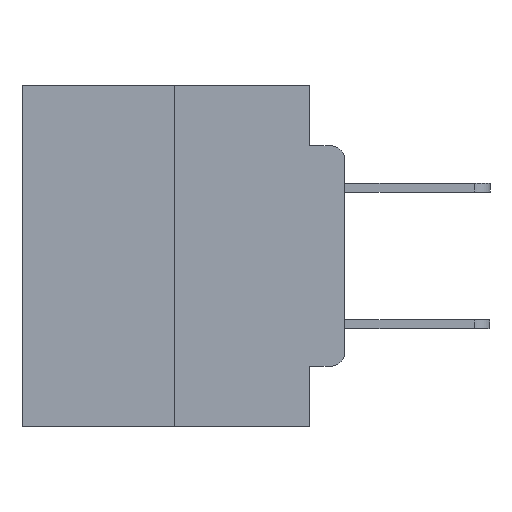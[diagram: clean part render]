
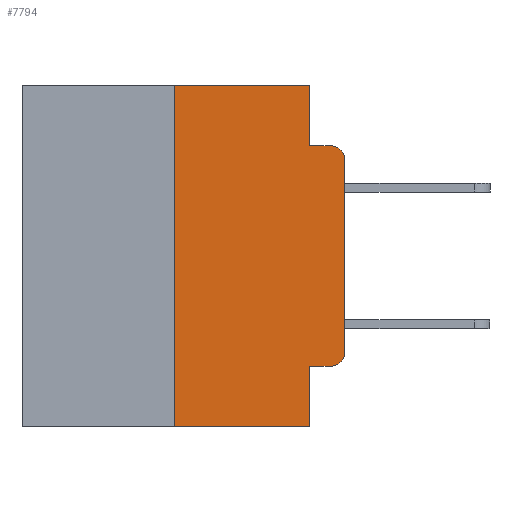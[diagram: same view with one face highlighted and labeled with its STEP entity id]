
A CAD part, left-side view. The second image highlights one B-rep face of the part: STEP entity #7794.
In plain terms, the highlighted planar face has unit normal (-1, 0, 0).
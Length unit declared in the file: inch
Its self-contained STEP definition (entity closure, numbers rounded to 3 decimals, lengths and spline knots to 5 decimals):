
#229 = VERTEX_POINT ( 'NONE', #24370 ) ;
#333 = DIRECTION ( 'NONE',  ( -1., 0., 0. ) ) ;
#425 = CARTESIAN_POINT ( 'NONE',  ( 0., 0.473, 0. ) ) ;
#692 = DIRECTION ( 'NONE',  ( -1., 0., 0. ) ) ;
#1464 = FACE_OUTER_BOUND ( 'NONE', #6110, .T. ) ;
#1516 = CARTESIAN_POINT ( 'NONE',  ( 0., 0.051, -0.0885 ) ) ;
#1519 = VERTEX_POINT ( 'NONE', #24135 ) ;
#2058 = ORIENTED_EDGE ( 'NONE', *, *, #5218, .F. ) ;
#2216 = VERTEX_POINT ( 'NONE', #14894 ) ;
#2325 = EDGE_CURVE ( 'NONE', #20849, #1519, #4652, .T. ) ;
#2396 = AXIS2_PLACEMENT_3D ( 'NONE', #13055, #333, #15138 ) ;
#3966 = LINE ( 'NONE', #7773, #14443 ) ;
#4499 = CARTESIAN_POINT ( 'NONE',  ( 0., 0.051, -0.4115 ) ) ;
#4652 = LINE ( 'NONE', #6540, #10197 ) ;
#5218 = EDGE_CURVE ( 'NONE', #9218, #19917, #16582, .T. ) ;
#5557 = VECTOR ( 'NONE', #22373, 39.37008 ) ;
#6054 = VECTOR ( 'NONE', #15220, 39.37008 ) ;
#6100 = CARTESIAN_POINT ( 'NONE',  ( 0., 0.473, 0. ) ) ;
#6110 = EDGE_LOOP ( 'NONE', ( #26407, #10629, #16791, #6409, #22850, #2058, #24161, #14549, #20001, #15845 ) ) ;
#6195 = DIRECTION ( 'NONE',  ( 0., 0., -1. ) ) ;
#6409 = ORIENTED_EDGE ( 'NONE', *, *, #2325, .F. ) ;
#6540 = CARTESIAN_POINT ( 'NONE',  ( 0., 0.051, 0. ) ) ;
#7129 = EDGE_CURVE ( 'NONE', #1519, #9947, #11082, .T. ) ;
#7773 = CARTESIAN_POINT ( 'NONE',  ( 0., 0.051, 0. ) ) ;
#7794 = ADVANCED_FACE ( 'NONE', ( #1464 ), #24679, .F. ) ;
#8178 = CARTESIAN_POINT ( 'NONE',  ( 0., 0.051, -0.4115 ) ) ;
#8709 = CARTESIAN_POINT ( 'NONE',  ( 0., 0.051, 0. ) ) ;
#9218 = VERTEX_POINT ( 'NONE', #23624 ) ;
#9471 = CARTESIAN_POINT ( 'NONE',  ( 0., 0., -0.1085 ) ) ;
#9864 = DIRECTION ( 'NONE',  ( 0., 0., -1. ) ) ;
#9947 = VERTEX_POINT ( 'NONE', #22607 ) ;
#10197 = VECTOR ( 'NONE', #10483, 39.37008 ) ;
#10483 = DIRECTION ( 'NONE',  ( 0., 0., -1. ) ) ;
#10629 = ORIENTED_EDGE ( 'NONE', *, *, #25618, .T. ) ;
#10925 = LINE ( 'NONE', #425, #6054 ) ;
#10948 = DIRECTION ( 'NONE',  ( 0., 0., 1. ) ) ;
#11082 = LINE ( 'NONE', #1516, #5557 ) ;
#11092 = LINE ( 'NONE', #16320, #15986 ) ;
#11131 = AXIS2_PLACEMENT_3D ( 'NONE', #6100, #18591, #6195 ) ;
#11850 = CARTESIAN_POINT ( 'NONE',  ( 0., 0.473, -0.5 ) ) ;
#12018 = EDGE_CURVE ( 'NONE', #229, #2216, #24056, .T. ) ;
#13055 = CARTESIAN_POINT ( 'NONE',  ( 0., 0.02, -0.3915 ) ) ;
#13382 = CARTESIAN_POINT ( 'NONE',  ( 0., 0.02, -0.1085 ) ) ;
#13975 = DIRECTION ( 'NONE',  ( 0., -1., 0. ) ) ;
#14443 = VECTOR ( 'NONE', #9864, 39.37008 ) ;
#14488 = CIRCLE ( 'NONE', #19791, 0.02 ) ;
#14549 = ORIENTED_EDGE ( 'NONE', *, *, #24588, .F. ) ;
#14894 = CARTESIAN_POINT ( 'NONE',  ( 0., 0., -0.3915 ) ) ;
#15100 = VECTOR ( 'NONE', #13975, 39.37008 ) ;
#15138 = DIRECTION ( 'NONE',  ( 0., 0., -1. ) ) ;
#15152 = CARTESIAN_POINT ( 'NONE',  ( 0., 0.25, 0. ) ) ;
#15220 = DIRECTION ( 'NONE',  ( 0., -1., 0. ) ) ;
#15232 = LINE ( 'NONE', #8178, #24816 ) ;
#15352 = EDGE_CURVE ( 'NONE', #17832, #229, #15232, .T. ) ;
#15465 = DIRECTION ( 'NONE',  ( 0., 0., -1. ) ) ;
#15573 = CARTESIAN_POINT ( 'NONE',  ( 0., 0.051, -0.5 ) ) ;
#15845 = ORIENTED_EDGE ( 'NONE', *, *, #12018, .T. ) ;
#15986 = VECTOR ( 'NONE', #22479, 39.37008 ) ;
#16320 = CARTESIAN_POINT ( 'NONE',  ( 0., 0., 0. ) ) ;
#16582 = LINE ( 'NONE', #15152, #21385 ) ;
#16791 = ORIENTED_EDGE ( 'NONE', *, *, #7129, .F. ) ;
#17832 = VERTEX_POINT ( 'NONE', #4499 ) ;
#18046 = CARTESIAN_POINT ( 'NONE',  ( 0., 0.25, 0. ) ) ;
#18591 = DIRECTION ( 'NONE',  ( 1., 0., 0. ) ) ;
#18739 = EDGE_CURVE ( 'NONE', #2216, #22602, #11092, .T. ) ;
#19791 = AXIS2_PLACEMENT_3D ( 'NONE', #13382, #692, #15465 ) ;
#19917 = VERTEX_POINT ( 'NONE', #18046 ) ;
#20001 = ORIENTED_EDGE ( 'NONE', *, *, #15352, .T. ) ;
#20849 = VERTEX_POINT ( 'NONE', #8709 ) ;
#21385 = VECTOR ( 'NONE', #10948, 39.37008 ) ;
#22373 = DIRECTION ( 'NONE',  ( 0., -1., 0. ) ) ;
#22479 = DIRECTION ( 'NONE',  ( 0., 0., 1. ) ) ;
#22551 = VERTEX_POINT ( 'NONE', #15573 ) ;
#22602 = VERTEX_POINT ( 'NONE', #9471 ) ;
#22607 = CARTESIAN_POINT ( 'NONE',  ( 0., 0.02, -0.0885 ) ) ;
#22850 = ORIENTED_EDGE ( 'NONE', *, *, #23150, .F. ) ;
#23150 = EDGE_CURVE ( 'NONE', #19917, #20849, #10925, .T. ) ;
#23624 = CARTESIAN_POINT ( 'NONE',  ( 0., 0.25, -0.5 ) ) ;
#24056 = CIRCLE ( 'NONE', #2396, 0.02 ) ;
#24135 = CARTESIAN_POINT ( 'NONE',  ( 0., 0.051, -0.0885 ) ) ;
#24161 = ORIENTED_EDGE ( 'NONE', *, *, #24574, .T. ) ;
#24370 = CARTESIAN_POINT ( 'NONE',  ( 0., 0.02, -0.4115 ) ) ;
#24574 = EDGE_CURVE ( 'NONE', #9218, #22551, #26625, .T. ) ;
#24588 = EDGE_CURVE ( 'NONE', #17832, #22551, #3966, .T. ) ;
#24679 = PLANE ( 'NONE',  #11131 ) ;
#24816 = VECTOR ( 'NONE', #26716, 39.37008 ) ;
#25618 = EDGE_CURVE ( 'NONE', #22602, #9947, #14488, .T. ) ;
#26407 = ORIENTED_EDGE ( 'NONE', *, *, #18739, .T. ) ;
#26625 = LINE ( 'NONE', #11850, #15100 ) ;
#26716 = DIRECTION ( 'NONE',  ( 0., -1., 0. ) ) ;
